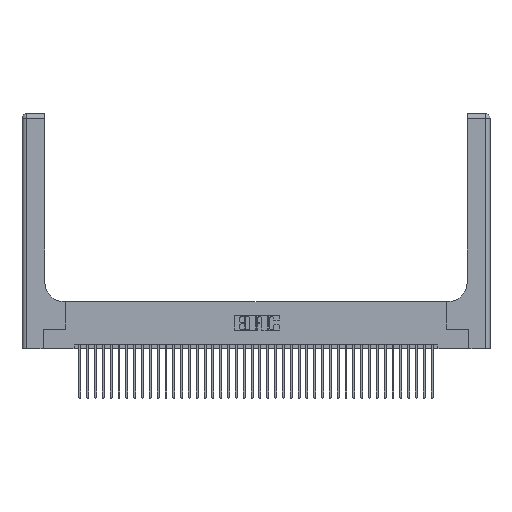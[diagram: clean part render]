
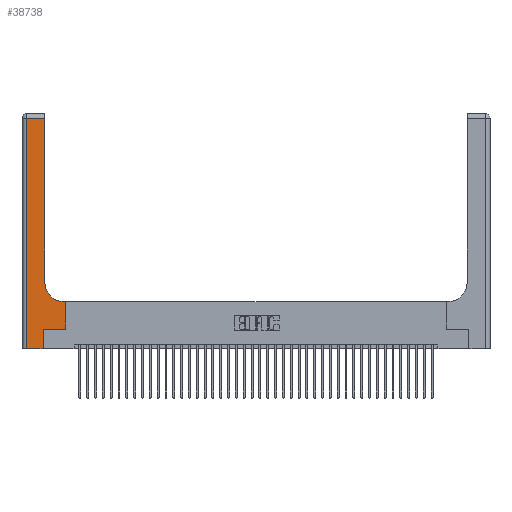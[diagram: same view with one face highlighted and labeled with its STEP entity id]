
A CAD part, top view. The second image highlights one B-rep face of the part: STEP entity #38738.
In plain terms, the highlighted planar face has unit normal (0, 0, 1).
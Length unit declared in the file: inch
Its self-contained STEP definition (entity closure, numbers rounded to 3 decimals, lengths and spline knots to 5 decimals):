
#451 = AXIS2_PLACEMENT_3D ( 'NONE', #11019, #16844, #37082 ) ;
#1127 = ORIENTED_EDGE ( 'NONE', *, *, #16776, .T. ) ;
#1335 = VERTEX_POINT ( 'NONE', #40036 ) ;
#1671 = DIRECTION ( 'NONE',  ( 1., 0., 0. ) ) ;
#1786 = VERTEX_POINT ( 'NONE', #5460 ) ;
#2575 = CARTESIAN_POINT ( 'NONE',  ( 0.06, 3., 0.37 ) ) ;
#3522 = CARTESIAN_POINT ( 'NONE',  ( 0.2915, 0.6, 0.37 ) ) ;
#5460 = CARTESIAN_POINT ( 'NONE',  ( 0.06, 2.94, 0.37 ) ) ;
#6300 = LINE ( 'NONE', #29939, #13739 ) ;
#6573 = PLANE ( 'NONE',  #18994 ) ;
#6696 = DIRECTION ( 'NONE',  ( 0., 0., -1. ) ) ;
#6796 = DIRECTION ( 'NONE',  ( -1., 0., 0. ) ) ;
#7086 = ORIENTED_EDGE ( 'NONE', *, *, #33964, .T. ) ;
#7743 = VERTEX_POINT ( 'NONE', #14122 ) ;
#8515 = VERTEX_POINT ( 'NONE', #12721 ) ;
#8906 = CARTESIAN_POINT ( 'NONE',  ( 0.06, 0., 0.37 ) ) ;
#9191 = CARTESIAN_POINT ( 'NONE',  ( 0.5585, 0.6, 0.37 ) ) ;
#9793 = LINE ( 'NONE', #39401, #31567 ) ;
#10567 = LINE ( 'NONE', #17419, #33741 ) ;
#11019 = CARTESIAN_POINT ( 'NONE',  ( 0.5415, 0.85, 0.37 ) ) ;
#11134 = ORIENTED_EDGE ( 'NONE', *, *, #30981, .T. ) ;
#11561 = FACE_OUTER_BOUND ( 'NONE', #36269, .T. ) ;
#12140 = DIRECTION ( 'NONE',  ( 0., 1., 0. ) ) ;
#12330 = VERTEX_POINT ( 'NONE', #15228 ) ;
#12416 = VERTEX_POINT ( 'NONE', #27756 ) ;
#12657 = EDGE_CURVE ( 'NONE', #1786, #40411, #29982, .T. ) ;
#12721 = CARTESIAN_POINT ( 'NONE',  ( 0.2915, 2.94, 0.37 ) ) ;
#13739 = VECTOR ( 'NONE', #12140, 39.37008 ) ;
#14122 = CARTESIAN_POINT ( 'NONE',  ( 0.5415, 0.6, 0.37 ) ) ;
#14403 = CARTESIAN_POINT ( 'NONE',  ( 0.269, 0., 0.37 ) ) ;
#15228 = CARTESIAN_POINT ( 'NONE',  ( 0.269, 0.25, 0.37 ) ) ;
#16776 = EDGE_CURVE ( 'NONE', #7743, #29350, #30631, .T. ) ;
#16844 = DIRECTION ( 'NONE',  ( 0., 0., -1. ) ) ;
#17419 = CARTESIAN_POINT ( 'NONE',  ( 0., 2.94, 0.37 ) ) ;
#17744 = EDGE_CURVE ( 'NONE', #29350, #8515, #6300, .T. ) ;
#18994 = AXIS2_PLACEMENT_3D ( 'NONE', #35275, #6696, #31869 ) ;
#20183 = LINE ( 'NONE', #14403, #28091 ) ;
#20669 = EDGE_CURVE ( 'NONE', #12416, #12330, #20183, .T. ) ;
#21824 = VECTOR ( 'NONE', #6796, 39.37008 ) ;
#22228 = ORIENTED_EDGE ( 'NONE', *, *, #17744, .T. ) ;
#23347 = DIRECTION ( 'NONE',  ( -1., 0., 0. ) ) ;
#23890 = EDGE_CURVE ( 'NONE', #12330, #1335, #33737, .T. ) ;
#26159 = ORIENTED_EDGE ( 'NONE', *, *, #20669, .T. ) ;
#27290 = LINE ( 'NONE', #40086, #40081 ) ;
#27756 = CARTESIAN_POINT ( 'NONE',  ( 0.269, 0., 0.37 ) ) ;
#27865 = VECTOR ( 'NONE', #35323, 39.37008 ) ;
#28091 = VECTOR ( 'NONE', #39736, 39.37008 ) ;
#29014 = CARTESIAN_POINT ( 'NONE',  ( 0.269, 0.25, 0.37 ) ) ;
#29350 = VERTEX_POINT ( 'NONE', #38227 ) ;
#29480 = ORIENTED_EDGE ( 'NONE', *, *, #23890, .T. ) ;
#29939 = CARTESIAN_POINT ( 'NONE',  ( 0.2915, 3., 0.37 ) ) ;
#29982 = LINE ( 'NONE', #2575, #38794 ) ;
#30631 = CIRCLE ( 'NONE', #451, 0.25 ) ;
#30981 = EDGE_CURVE ( 'NONE', #32897, #7743, #32163, .T. ) ;
#31567 = VECTOR ( 'NONE', #1671, 39.37008 ) ;
#31869 = DIRECTION ( 'NONE',  ( -1., 0., 0. ) ) ;
#32163 = LINE ( 'NONE', #3522, #21824 ) ;
#32897 = VERTEX_POINT ( 'NONE', #9191 ) ;
#33737 = LINE ( 'NONE', #29014, #27865 ) ;
#33741 = VECTOR ( 'NONE', #23347, 39.37008 ) ;
#33964 = EDGE_CURVE ( 'NONE', #8515, #1786, #10567, .T. ) ;
#34276 = ORIENTED_EDGE ( 'NONE', *, *, #12657, .T. ) ;
#34609 = EDGE_CURVE ( 'NONE', #1335, #32897, #27290, .T. ) ;
#34954 = ORIENTED_EDGE ( 'NONE', *, *, #34609, .T. ) ;
#35275 = CARTESIAN_POINT ( 'NONE',  ( 0., 3., 0.37 ) ) ;
#35323 = DIRECTION ( 'NONE',  ( 1., 0., 0. ) ) ;
#36269 = EDGE_LOOP ( 'NONE', ( #22228, #7086, #34276, #38121, #26159, #29480, #34954, #11134, #1127 ) ) ;
#36956 = EDGE_CURVE ( 'NONE', #40411, #12416, #9793, .T. ) ;
#37082 = DIRECTION ( 'NONE',  ( 1., 0., 0. ) ) ;
#38121 = ORIENTED_EDGE ( 'NONE', *, *, #36956, .T. ) ;
#38227 = CARTESIAN_POINT ( 'NONE',  ( 0.2915, 0.85, 0.37 ) ) ;
#38738 = ADVANCED_FACE ( 'NONE', ( #11561 ), #6573, .F. ) ;
#38794 = VECTOR ( 'NONE', #38900, 39.37008 ) ;
#38900 = DIRECTION ( 'NONE',  ( 0., -1., 0. ) ) ;
#39401 = CARTESIAN_POINT ( 'NONE',  ( 0., 0., 0.37 ) ) ;
#39654 = DIRECTION ( 'NONE',  ( 0., 1., 0. ) ) ;
#39736 = DIRECTION ( 'NONE',  ( 0., 1., 0. ) ) ;
#40036 = CARTESIAN_POINT ( 'NONE',  ( 0.5585, 0.25, 0.37 ) ) ;
#40081 = VECTOR ( 'NONE', #39654, 39.37008 ) ;
#40086 = CARTESIAN_POINT ( 'NONE',  ( 0.5585, 0.25, 0.37 ) ) ;
#40411 = VERTEX_POINT ( 'NONE', #8906 ) ;
